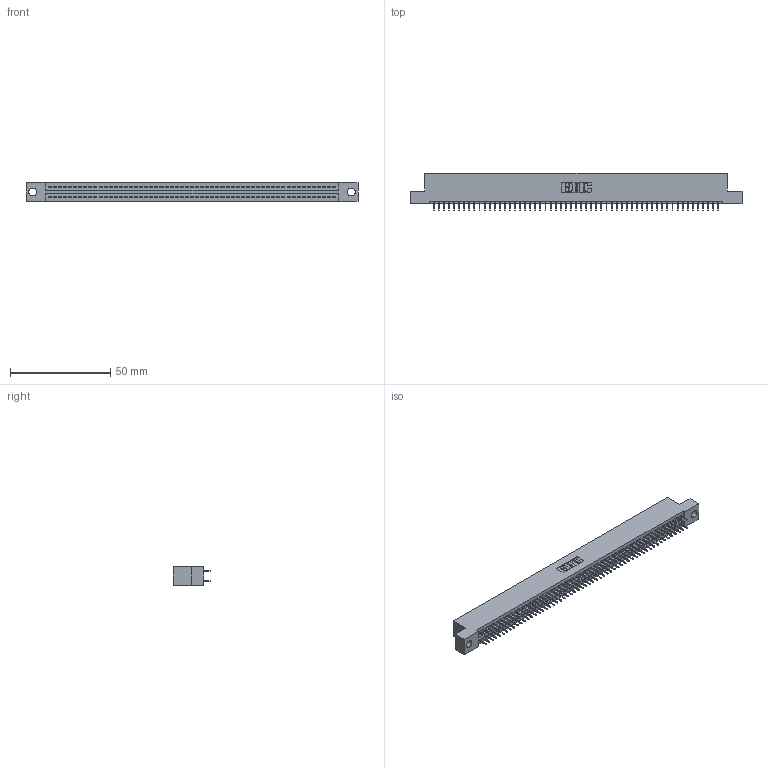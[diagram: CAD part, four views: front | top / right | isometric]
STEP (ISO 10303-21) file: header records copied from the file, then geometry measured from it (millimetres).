
FILE_DESCRIPTION (( 'STEP AP203' ), '1' );
FILE_NAME ('345-114-525-204.STEP', '2020-09-21T22:20:10', ( '' ), ( '' ), 'SwSTEP 2.0', 'SolidWorks 2020', '' );
FILE_SCHEMA (( 'CONFIG_CONTROL_DESIGN' ));
Length unit declared in the file: inch
Products named in the file (3): 345-292-001_345-293-125; 345-114-525-204; 345 Part_Flush Mounting Lugs - 0.156 Dia-TH
Assembly tree (115 placements, depth 2):
  345-114-525-204
    345 Part_Flush Mounting Lugs - 0.156 Dia-TH
    345-292-001_345-293-125  x114
Bounding box: 165.99 x 18.72 x 9.4 mm (x, y, z)
Volume: 15988.1 mm3; surface area: 23173.3 mm2
Topology: 115 solids, 115 shells, 6282 faces, 17783 edges, 11398 vertices
Faces by surface type: plane 4526, cylinder 1756
Entity records: 42781 total; most frequent: CARTESIAN_POINT 7156, ORIENTED_EDGE 7090, DIRECTION 6293, EDGE_CURVE 3545, VECTOR 3189, LINE 3189, VERTEX_POINT 2358, AXIS2_PLACEMENT_3D 1552
